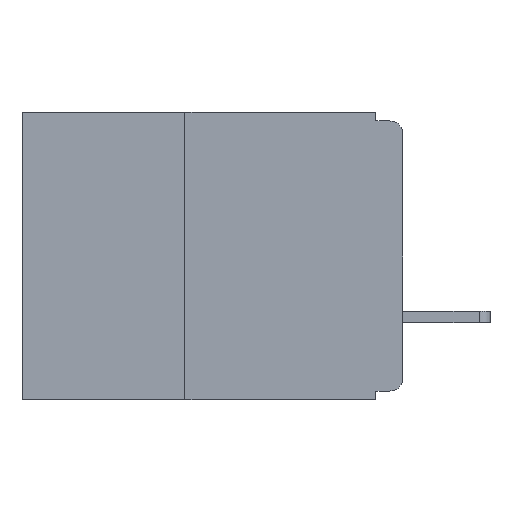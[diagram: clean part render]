
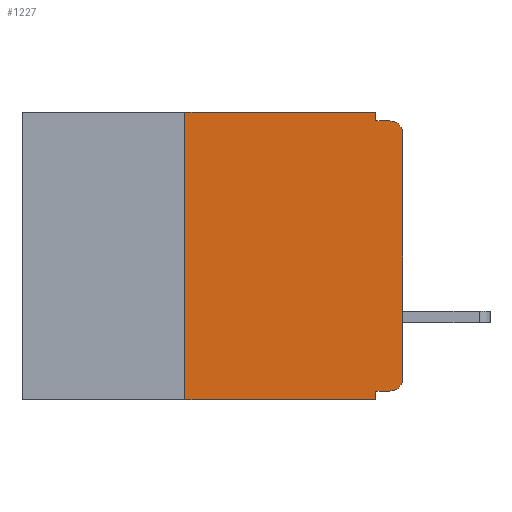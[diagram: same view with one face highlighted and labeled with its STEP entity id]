
A CAD part, left-side view. The second image highlights one B-rep face of the part: STEP entity #1227.
In plain terms, the highlighted planar face has unit normal (-1, 0, 0).
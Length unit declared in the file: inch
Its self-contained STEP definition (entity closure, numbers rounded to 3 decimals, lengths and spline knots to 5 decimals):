
#155 = LINE ( 'NONE', #3869, #10711 ) ;
#232 = DIRECTION ( 'NONE',  ( 0., 0., -1. ) ) ;
#260 = VECTOR ( 'NONE', #4694, 39.37008 ) ;
#388 = ORIENTED_EDGE ( 'NONE', *, *, #10315, .F. ) ;
#393 = DIRECTION ( 'NONE',  ( 0., -1., 0. ) ) ;
#644 = VERTEX_POINT ( 'NONE', #3346 ) ;
#703 = DIRECTION ( 'NONE',  ( -1., 0., 0. ) ) ;
#968 = ORIENTED_EDGE ( 'NONE', *, *, #12385, .T. ) ;
#1115 = DIRECTION ( 'NONE',  ( 0., 0., -1. ) ) ;
#1227 = ADVANCED_FACE ( 'NONE', ( #2716 ), #15182, .F. ) ;
#1308 = EDGE_CURVE ( 'NONE', #15508, #6260, #1336, .T. ) ;
#1336 = LINE ( 'NONE', #12254, #4766 ) ;
#1461 = ORIENTED_EDGE ( 'NONE', *, *, #9216, .F. ) ;
#1652 = VECTOR ( 'NONE', #393, 39.37008 ) ;
#1690 = CIRCLE ( 'NONE', #2013, 0.015 ) ;
#1975 = ORIENTED_EDGE ( 'NONE', *, *, #1308, .T. ) ;
#2013 = AXIS2_PLACEMENT_3D ( 'NONE', #15379, #703, #16191 ) ;
#2127 = EDGE_CURVE ( 'NONE', #15222, #13230, #155, .T. ) ;
#2144 = ORIENTED_EDGE ( 'NONE', *, *, #9458, .T. ) ;
#2424 = DIRECTION ( 'NONE',  ( 0., 0., 1. ) ) ;
#2488 = CARTESIAN_POINT ( 'NONE',  ( 0., 0.015, -0.32 ) ) ;
#2701 = VERTEX_POINT ( 'NONE', #14796 ) ;
#2716 = FACE_OUTER_BOUND ( 'NONE', #8699, .T. ) ;
#3031 = ORIENTED_EDGE ( 'NONE', *, *, #3990, .T. ) ;
#3223 = VECTOR ( 'NONE', #2424, 39.37008 ) ;
#3346 = CARTESIAN_POINT ( 'NONE',  ( 0., 0.031, 0. ) ) ;
#3541 = DIRECTION ( 'NONE',  ( 0., 0., 1. ) ) ;
#3869 = CARTESIAN_POINT ( 'NONE',  ( 0., 0., -0.32 ) ) ;
#3990 = EDGE_CURVE ( 'NONE', #15222, #14824, #1690, .T. ) ;
#4694 = DIRECTION ( 'NONE',  ( 0., -1., 0. ) ) ;
#4766 = VECTOR ( 'NONE', #16966, 39.37008 ) ;
#4795 = VECTOR ( 'NONE', #3541, 39.37008 ) ;
#6260 = VERTEX_POINT ( 'NONE', #10372 ) ;
#6289 = VERTEX_POINT ( 'NONE', #11915 ) ;
#6491 = DIRECTION ( 'NONE',  ( 0., 0., -1. ) ) ;
#6614 = DIRECTION ( 'NONE',  ( 1., 0., 0. ) ) ;
#6688 = CARTESIAN_POINT ( 'NONE',  ( 0., 0.25, -0.33 ) ) ;
#6723 = CARTESIAN_POINT ( 'NONE',  ( 0., 0.437, 0. ) ) ;
#6819 = CIRCLE ( 'NONE', #17394, 0.015 ) ;
#6991 = CARTESIAN_POINT ( 'NONE',  ( 0., 0.25, 0. ) ) ;
#7329 = VECTOR ( 'NONE', #8829, 39.37008 ) ;
#7985 = EDGE_CURVE ( 'NONE', #10705, #644, #13017, .T. ) ;
#8505 = LINE ( 'NONE', #8878, #15477 ) ;
#8699 = EDGE_LOOP ( 'NONE', ( #968, #2144, #1461, #11104, #9684, #12518, #1975, #388, #9723, #3031 ) ) ;
#8704 = CARTESIAN_POINT ( 'NONE',  ( 0., 0., -0.305 ) ) ;
#8829 = DIRECTION ( 'NONE',  ( 0., 0., -1. ) ) ;
#8878 = CARTESIAN_POINT ( 'NONE',  ( 0., 0.031, 0. ) ) ;
#9157 = AXIS2_PLACEMENT_3D ( 'NONE', #6723, #6614, #6491 ) ;
#9216 = EDGE_CURVE ( 'NONE', #6289, #12325, #15359, .T. ) ;
#9458 = EDGE_CURVE ( 'NONE', #2701, #12325, #6819, .T. ) ;
#9684 = ORIENTED_EDGE ( 'NONE', *, *, #7985, .F. ) ;
#9714 = DIRECTION ( 'NONE',  ( -1., 0., 0. ) ) ;
#9723 = ORIENTED_EDGE ( 'NONE', *, *, #2127, .F. ) ;
#10236 = CARTESIAN_POINT ( 'NONE',  ( 0., 0.031, -0.33 ) ) ;
#10315 = EDGE_CURVE ( 'NONE', #13230, #6260, #11060, .T. ) ;
#10372 = CARTESIAN_POINT ( 'NONE',  ( 0., 0.031, -0.33 ) ) ;
#10439 = CARTESIAN_POINT ( 'NONE',  ( 0., 0.437, 0. ) ) ;
#10579 = CARTESIAN_POINT ( 'NONE',  ( 0., 0.015, -0.01 ) ) ;
#10705 = VERTEX_POINT ( 'NONE', #6991 ) ;
#10711 = VECTOR ( 'NONE', #15087, 39.37008 ) ;
#10758 = CARTESIAN_POINT ( 'NONE',  ( 0., 0., 0. ) ) ;
#11060 = LINE ( 'NONE', #10236, #7329 ) ;
#11104 = ORIENTED_EDGE ( 'NONE', *, *, #13692, .F. ) ;
#11593 = CARTESIAN_POINT ( 'NONE',  ( 0., 0.031, -0.32 ) ) ;
#11859 = EDGE_CURVE ( 'NONE', #15508, #10705, #14050, .T. ) ;
#11896 = CARTESIAN_POINT ( 'NONE',  ( 0., 0.25, -0.33 ) ) ;
#11915 = CARTESIAN_POINT ( 'NONE',  ( 0., 0.031, -0.01 ) ) ;
#12254 = CARTESIAN_POINT ( 'NONE',  ( 0., 0.437, -0.33 ) ) ;
#12325 = VERTEX_POINT ( 'NONE', #10579 ) ;
#12385 = EDGE_CURVE ( 'NONE', #14824, #2701, #15993, .T. ) ;
#12518 = ORIENTED_EDGE ( 'NONE', *, *, #11859, .F. ) ;
#13017 = LINE ( 'NONE', #10439, #1652 ) ;
#13139 = CARTESIAN_POINT ( 'NONE',  ( 0., 0., -0.01 ) ) ;
#13230 = VERTEX_POINT ( 'NONE', #11593 ) ;
#13692 = EDGE_CURVE ( 'NONE', #644, #6289, #8505, .T. ) ;
#14050 = LINE ( 'NONE', #6688, #3223 ) ;
#14796 = CARTESIAN_POINT ( 'NONE',  ( 0., 0., -0.025 ) ) ;
#14824 = VERTEX_POINT ( 'NONE', #8704 ) ;
#15087 = DIRECTION ( 'NONE',  ( 0., 1., 0. ) ) ;
#15182 = PLANE ( 'NONE',  #9157 ) ;
#15222 = VERTEX_POINT ( 'NONE', #2488 ) ;
#15359 = LINE ( 'NONE', #13139, #260 ) ;
#15379 = CARTESIAN_POINT ( 'NONE',  ( 0., 0.015, -0.305 ) ) ;
#15477 = VECTOR ( 'NONE', #232, 39.37008 ) ;
#15508 = VERTEX_POINT ( 'NONE', #11896 ) ;
#15993 = LINE ( 'NONE', #10758, #4795 ) ;
#16191 = DIRECTION ( 'NONE',  ( 0., 0., -1. ) ) ;
#16966 = DIRECTION ( 'NONE',  ( 0., -1., 0. ) ) ;
#17394 = AXIS2_PLACEMENT_3D ( 'NONE', #17963, #9714, #1115 ) ;
#17963 = CARTESIAN_POINT ( 'NONE',  ( 0., 0.015, -0.025 ) ) ;
